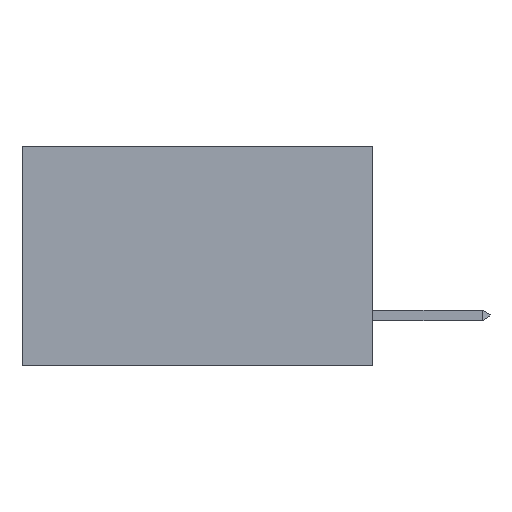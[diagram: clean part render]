
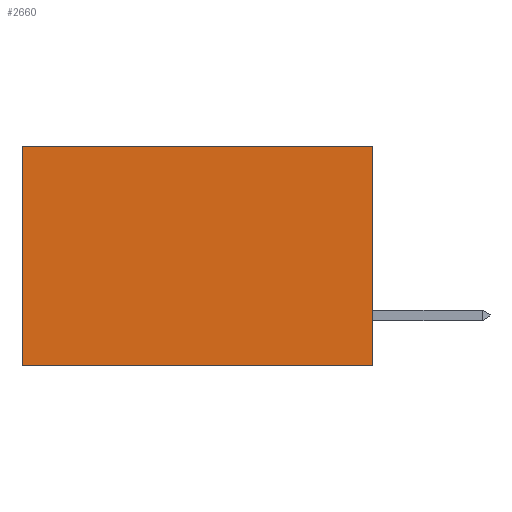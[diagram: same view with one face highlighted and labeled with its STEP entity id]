
A CAD part, left-side view. The second image highlights one B-rep face of the part: STEP entity #2660.
In plain terms, the highlighted planar face has unit normal (-1, 0, 0).
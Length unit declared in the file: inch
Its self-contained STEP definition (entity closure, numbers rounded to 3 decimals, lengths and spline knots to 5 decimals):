
#2660 = ADVANCED_FACE ( 'NONE', ( #15042 ), #19325, .F. ) ;
#3614 = VECTOR ( 'NONE', #27411, 39.37008 ) ;
#4267 = DIRECTION ( 'NONE',  ( 0., 1., 0. ) ) ;
#5215 = CARTESIAN_POINT ( 'NONE',  ( 0.277, 0.59, -0.37 ) ) ;
#6300 = VERTEX_POINT ( 'NONE', #18849 ) ;
#8499 = VECTOR ( 'NONE', #4267, 39.37008 ) ;
#8837 = EDGE_LOOP ( 'NONE', ( #14737, #16450, #13116, #10129 ) ) ;
#9437 = VECTOR ( 'NONE', #20202, 39.37008 ) ;
#9822 = CARTESIAN_POINT ( 'NONE',  ( 0.277, 0., -0.37 ) ) ;
#10129 = ORIENTED_EDGE ( 'NONE', *, *, #16737, .T. ) ;
#10947 = VERTEX_POINT ( 'NONE', #24816 ) ;
#11346 = VECTOR ( 'NONE', #18051, 39.37008 ) ;
#13116 = ORIENTED_EDGE ( 'NONE', *, *, #28620, .F. ) ;
#14737 = ORIENTED_EDGE ( 'NONE', *, *, #21271, .T. ) ;
#15042 = FACE_OUTER_BOUND ( 'NONE', #8837, .T. ) ;
#15345 = LINE ( 'NONE', #19571, #8499 ) ;
#16258 = LINE ( 'NONE', #9822, #9437 ) ;
#16450 = ORIENTED_EDGE ( 'NONE', *, *, #19792, .F. ) ;
#16737 = EDGE_CURVE ( 'NONE', #32456, #10947, #15345, .T. ) ;
#17280 = LINE ( 'NONE', #24900, #3614 ) ;
#17454 = CARTESIAN_POINT ( 'NONE',  ( 0.277, 0., 0. ) ) ;
#18051 = DIRECTION ( 'NONE',  ( 0., 0., -1. ) ) ;
#18849 = CARTESIAN_POINT ( 'NONE',  ( 0.277, 0.59, -0.37 ) ) ;
#18990 = LINE ( 'NONE', #5215, #11346 ) ;
#19167 = DIRECTION ( 'NONE',  ( 1., 0., 0. ) ) ;
#19325 = PLANE ( 'NONE',  #23925 ) ;
#19571 = CARTESIAN_POINT ( 'NONE',  ( 0.277, 0., 0. ) ) ;
#19792 = EDGE_CURVE ( 'NONE', #22163, #6300, #16258, .T. ) ;
#20202 = DIRECTION ( 'NONE',  ( 0., 1., 0. ) ) ;
#21271 = EDGE_CURVE ( 'NONE', #10947, #6300, #18990, .T. ) ;
#22163 = VERTEX_POINT ( 'NONE', #31564 ) ;
#22221 = CARTESIAN_POINT ( 'NONE',  ( 0.277, 0., -0.37 ) ) ;
#22805 = DIRECTION ( 'NONE',  ( 0., 0., -1. ) ) ;
#23925 = AXIS2_PLACEMENT_3D ( 'NONE', #22221, #19167, #22805 ) ;
#24816 = CARTESIAN_POINT ( 'NONE',  ( 0.277, 0.59, 0. ) ) ;
#24900 = CARTESIAN_POINT ( 'NONE',  ( 0.277, 0., -0.37 ) ) ;
#27411 = DIRECTION ( 'NONE',  ( 0., 0., -1. ) ) ;
#28620 = EDGE_CURVE ( 'NONE', #32456, #22163, #17280, .T. ) ;
#31564 = CARTESIAN_POINT ( 'NONE',  ( 0.277, 0., -0.37 ) ) ;
#32456 = VERTEX_POINT ( 'NONE', #17454 ) ;
